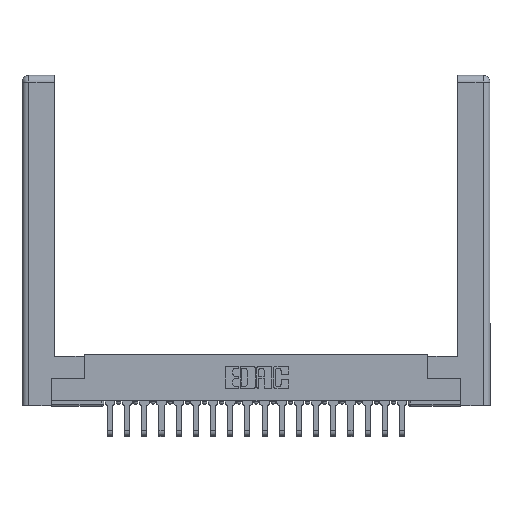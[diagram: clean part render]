
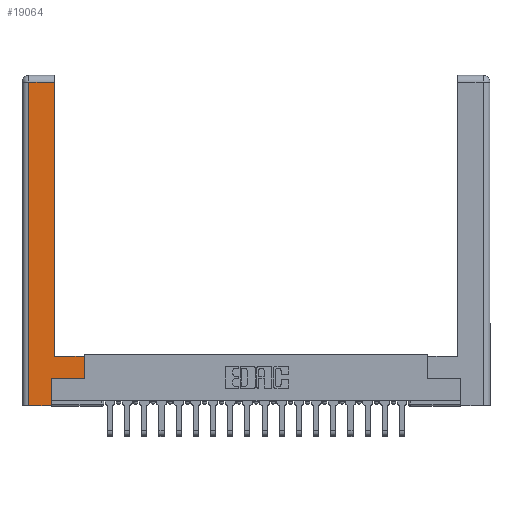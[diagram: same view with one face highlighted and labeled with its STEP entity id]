
A CAD part, top view. The second image highlights one B-rep face of the part: STEP entity #19064.
In plain terms, the highlighted planar face has unit normal (0, 0, 1).
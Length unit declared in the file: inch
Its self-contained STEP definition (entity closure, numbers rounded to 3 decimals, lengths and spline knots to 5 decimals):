
#161 = CARTESIAN_POINT ( 'NONE',  ( 0.0615, 2.94, 0. ) ) ;
#503 = CARTESIAN_POINT ( 'NONE',  ( 0.295, 3., 0. ) ) ;
#1430 = VERTEX_POINT ( 'NONE', #20355 ) ;
#2448 = LINE ( 'NONE', #9691, #20232 ) ;
#2757 = CARTESIAN_POINT ( 'NONE',  ( 0.565, 0.245, 0. ) ) ;
#2989 = LINE ( 'NONE', #9669, #11075 ) ;
#3970 = AXIS2_PLACEMENT_3D ( 'NONE', #20333, #16928, #11351 ) ;
#4016 = DIRECTION ( 'NONE',  ( 0., 1., 0. ) ) ;
#4163 = VECTOR ( 'NONE', #4016, 39.37008 ) ;
#4173 = CARTESIAN_POINT ( 'NONE',  ( 0.0615, 0., 0. ) ) ;
#4377 = VECTOR ( 'NONE', #22369, 39.37008 ) ;
#5258 = LINE ( 'NONE', #7245, #5302 ) ;
#5302 = VECTOR ( 'NONE', #14604, 39.37008 ) ;
#5490 = EDGE_CURVE ( 'NONE', #5917, #21626, #2448, .T. ) ;
#5917 = VERTEX_POINT ( 'NONE', #13271 ) ;
#5994 = CARTESIAN_POINT ( 'NONE',  ( 0.565, 0.245, 0. ) ) ;
#6452 = VECTOR ( 'NONE', #22437, 39.37008 ) ;
#6557 = VERTEX_POINT ( 'NONE', #22572 ) ;
#7245 = CARTESIAN_POINT ( 'NONE',  ( 0.265, 0.245, 0. ) ) ;
#7282 = VERTEX_POINT ( 'NONE', #4173 ) ;
#7644 = CARTESIAN_POINT ( 'NONE',  ( 0.295, 0.45, 0. ) ) ;
#7870 = EDGE_CURVE ( 'NONE', #21626, #8954, #14531, .T. ) ;
#8347 = CARTESIAN_POINT ( 'NONE',  ( 0.265, 0., 0. ) ) ;
#8925 = DIRECTION ( 'NONE',  ( -1., 0., 0. ) ) ;
#8954 = VERTEX_POINT ( 'NONE', #19682 ) ;
#9276 = LINE ( 'NONE', #161, #16119 ) ;
#9669 = CARTESIAN_POINT ( 'NONE',  ( 0.0615, 0., 0. ) ) ;
#9691 = CARTESIAN_POINT ( 'NONE',  ( 0.295, 0.45, 0. ) ) ;
#10062 = FACE_OUTER_BOUND ( 'NONE', #13515, .T. ) ;
#10103 = LINE ( 'NONE', #8347, #17444 ) ;
#10126 = DIRECTION ( 'NONE',  ( 0., -1., 0. ) ) ;
#10534 = EDGE_CURVE ( 'NONE', #14989, #5917, #20569, .T. ) ;
#11075 = VECTOR ( 'NONE', #10126, 39.37008 ) ;
#11310 = ORIENTED_EDGE ( 'NONE', *, *, #22930, .T. ) ;
#11351 = DIRECTION ( 'NONE',  ( -1., 0., 0. ) ) ;
#11504 = DIRECTION ( 'NONE',  ( 1., 0., 0. ) ) ;
#11993 = ORIENTED_EDGE ( 'NONE', *, *, #15600, .T. ) ;
#13117 = CARTESIAN_POINT ( 'NONE',  ( 0.265, 0.245, 0. ) ) ;
#13181 = DIRECTION ( 'NONE',  ( -1., 0., 0. ) ) ;
#13271 = CARTESIAN_POINT ( 'NONE',  ( 0.565, 0.45, 0. ) ) ;
#13515 = EDGE_LOOP ( 'NONE', ( #17935, #15388, #22857, #11310, #11993, #15503, #14297, #15602 ) ) ;
#14297 = ORIENTED_EDGE ( 'NONE', *, *, #10534, .T. ) ;
#14531 = LINE ( 'NONE', #503, #4163 ) ;
#14604 = DIRECTION ( 'NONE',  ( 0., 1., 0. ) ) ;
#14989 = VERTEX_POINT ( 'NONE', #5994 ) ;
#15283 = EDGE_CURVE ( 'NONE', #8954, #6557, #9276, .T. ) ;
#15388 = ORIENTED_EDGE ( 'NONE', *, *, #15283, .T. ) ;
#15503 = ORIENTED_EDGE ( 'NONE', *, *, #22490, .T. ) ;
#15572 = CARTESIAN_POINT ( 'NONE',  ( 0.565, 0.45, 0. ) ) ;
#15600 = EDGE_CURVE ( 'NONE', #1430, #17267, #5258, .T. ) ;
#15602 = ORIENTED_EDGE ( 'NONE', *, *, #5490, .T. ) ;
#16119 = VECTOR ( 'NONE', #8925, 39.37008 ) ;
#16711 = PLANE ( 'NONE',  #3970 ) ;
#16882 = LINE ( 'NONE', #2757, #4377 ) ;
#16928 = DIRECTION ( 'NONE',  ( 0., 0., -1. ) ) ;
#17267 = VERTEX_POINT ( 'NONE', #13117 ) ;
#17444 = VECTOR ( 'NONE', #11504, 39.37008 ) ;
#17935 = ORIENTED_EDGE ( 'NONE', *, *, #7870, .T. ) ;
#19064 = ADVANCED_FACE ( 'NONE', ( #10062 ), #16711, .F. ) ;
#19682 = CARTESIAN_POINT ( 'NONE',  ( 0.295, 2.94, 0. ) ) ;
#20232 = VECTOR ( 'NONE', #13181, 39.37008 ) ;
#20333 = CARTESIAN_POINT ( 'NONE',  ( 0., 0., 0. ) ) ;
#20355 = CARTESIAN_POINT ( 'NONE',  ( 0.265, 0., 0. ) ) ;
#20569 = LINE ( 'NONE', #15572, #6452 ) ;
#21315 = EDGE_CURVE ( 'NONE', #6557, #7282, #2989, .T. ) ;
#21626 = VERTEX_POINT ( 'NONE', #7644 ) ;
#22369 = DIRECTION ( 'NONE',  ( 1., 0., 0. ) ) ;
#22437 = DIRECTION ( 'NONE',  ( 0., 1., 0. ) ) ;
#22490 = EDGE_CURVE ( 'NONE', #17267, #14989, #16882, .T. ) ;
#22572 = CARTESIAN_POINT ( 'NONE',  ( 0.0615, 2.94, 0. ) ) ;
#22857 = ORIENTED_EDGE ( 'NONE', *, *, #21315, .T. ) ;
#22930 = EDGE_CURVE ( 'NONE', #7282, #1430, #10103, .T. ) ;
